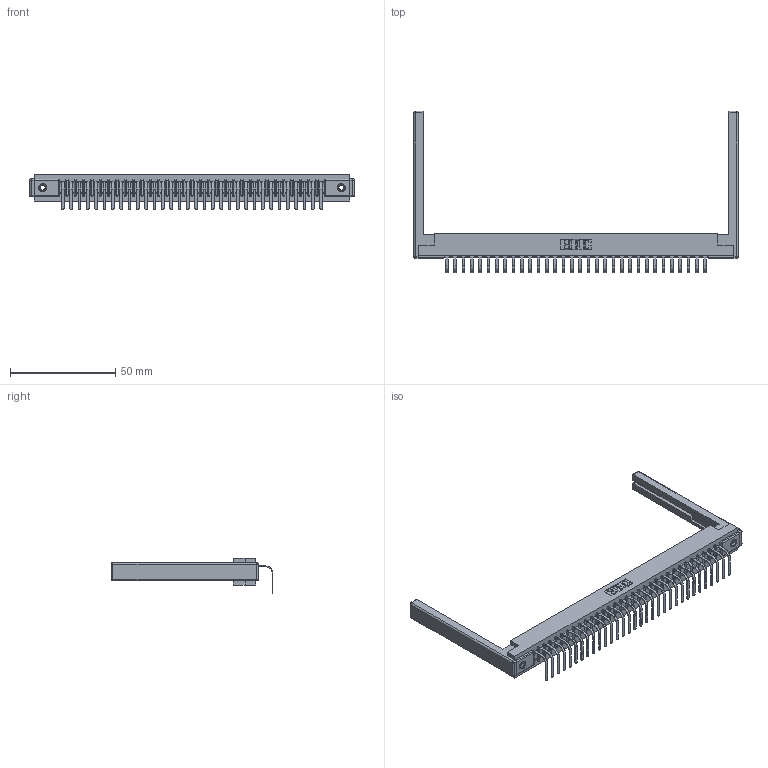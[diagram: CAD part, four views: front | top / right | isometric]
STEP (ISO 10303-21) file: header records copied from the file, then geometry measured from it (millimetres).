
FILE_DESCRIPTION (( 'STEP AP203' ), '1' );
FILE_NAME ('357-032-558-168.STEP', '2022-07-13T19:28:09', ( '' ), ( '' ), 'SwSTEP 2.0', 'SolidWorks 2020', '' );
FILE_SCHEMA (( 'CONFIG_CONTROL_DESIGN' ));
Length unit declared in the file: inch
Products named in the file (5): 357-032-558-168; 307-220-068; 307 Part_.156 Dia Mounting Holes; 345-250-001_345-250-001-102; 307-290-001_558 - 2 (Single)
Assembly tree (37 placements, depth 2):
  357-032-558-168
    307 Part_.156 Dia Mounting Holes
    307-290-001_558 - 2 (Single)  x32
    307-220-068  x2
    345-250-001_345-250-001-102  x2
Bounding box: 154.23 x 76.75 x 16.8 mm (x, y, z)
Volume: 20477.4 mm3; surface area: 21841 mm2
Topology: 37 solids, 37 shells, 2225 faces, 6281 edges, 4034 vertices
Faces by surface type: plane 1406, cylinder 729, sphere 74, cone 12, torus 4
Entity records: 31529 total; most frequent: CARTESIAN_POINT 5273, ORIENTED_EDGE 5248, DIRECTION 5152, EDGE_CURVE 2624, LINE 2006, VECTOR 2006, VERTEX_POINT 1694, AXIS2_PLACEMENT_3D 1573
